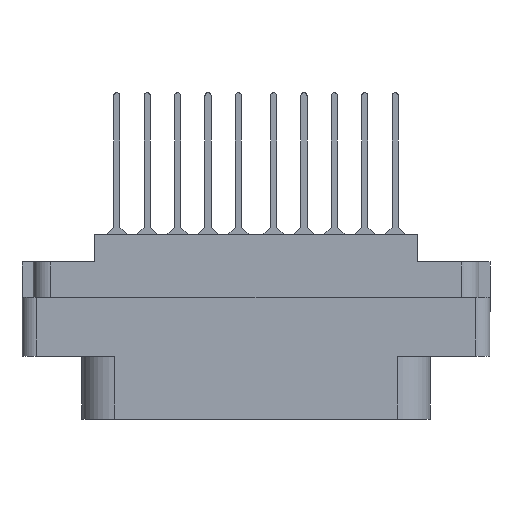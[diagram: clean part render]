
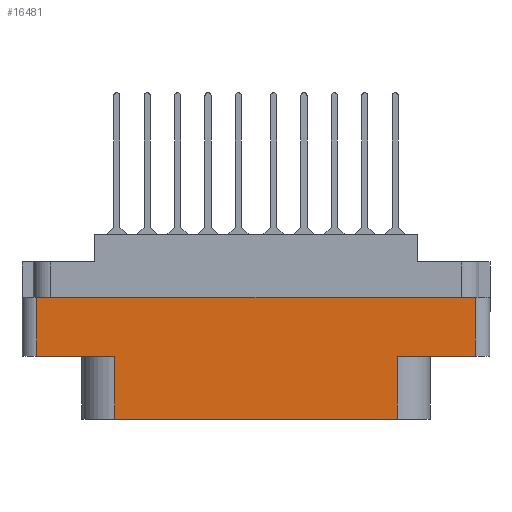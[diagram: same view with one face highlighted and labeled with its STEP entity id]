
A CAD part, front view. The second image highlights one B-rep face of the part: STEP entity #16481.
In plain terms, the highlighted planar face has unit normal (0, -1, 0).
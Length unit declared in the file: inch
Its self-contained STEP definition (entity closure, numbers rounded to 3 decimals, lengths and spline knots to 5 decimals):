
#424 = VECTOR ( 'NONE', #13086, 39.37008 ) ;
#2172 = CARTESIAN_POINT ( 'NONE',  ( 0.938, -0.438, -0.52 ) ) ;
#2329 = CARTESIAN_POINT ( 'NONE',  ( -0.604, -0.438, -0.789 ) ) ;
#3349 = LINE ( 'NONE', #35935, #7940 ) ;
#3606 = EDGE_CURVE ( 'NONE', #11798, #6598, #30297, .T. ) ;
#4166 = CARTESIAN_POINT ( 'NONE',  ( -0.938, -0.438, -0.789 ) ) ;
#5817 = VECTOR ( 'NONE', #22901, 39.37008 ) ;
#6598 = VERTEX_POINT ( 'NONE', #17969 ) ;
#6996 = LINE ( 'NONE', #27918, #11958 ) ;
#7242 = FACE_OUTER_BOUND ( 'NONE', #15127, .T. ) ;
#7872 = VERTEX_POINT ( 'NONE', #2329 ) ;
#7940 = VECTOR ( 'NONE', #24107, 39.37008 ) ;
#8310 = VECTOR ( 'NONE', #18949, 39.37008 ) ;
#10467 = DIRECTION ( 'NONE',  ( 1., 0., 0. ) ) ;
#10650 = DIRECTION ( 'NONE',  ( 1., 0., 0. ) ) ;
#11186 = LINE ( 'NONE', #19456, #34420 ) ;
#11798 = VERTEX_POINT ( 'NONE', #2172 ) ;
#11958 = VECTOR ( 'NONE', #10467, 39.37008 ) ;
#12614 = DIRECTION ( 'NONE',  ( 0., 0., -1. ) ) ;
#13086 = DIRECTION ( 'NONE',  ( 0., 0., -1. ) ) ;
#13253 = EDGE_CURVE ( 'NONE', #30960, #36560, #23623, .T. ) ;
#13269 = ORIENTED_EDGE ( 'NONE', *, *, #32429, .T. ) ;
#15127 = EDGE_LOOP ( 'NONE', ( #34025, #35011, #32678, #32936, #24844, #15879, #19700, #13269 ) ) ;
#15879 = ORIENTED_EDGE ( 'NONE', *, *, #31851, .T. ) ;
#16081 = VECTOR ( 'NONE', #28168, 39.37008 ) ;
#16481 = ADVANCED_FACE ( 'NONE', ( #7242 ), #27015, .T. ) ;
#17959 = VECTOR ( 'NONE', #33594, 39.37008 ) ;
#17969 = CARTESIAN_POINT ( 'NONE',  ( 0.604, -0.438, -0.52 ) ) ;
#18949 = DIRECTION ( 'NONE',  ( 0., 0., 1. ) ) ;
#19183 = CARTESIAN_POINT ( 'NONE',  ( 0.938, -0.438, -0.268 ) ) ;
#19456 = CARTESIAN_POINT ( 'NONE',  ( -1., -0.438, -0.789 ) ) ;
#19700 = ORIENTED_EDGE ( 'NONE', *, *, #3606, .F. ) ;
#21545 = CARTESIAN_POINT ( 'NONE',  ( 0.604, -0.438, -0.789 ) ) ;
#21825 = EDGE_CURVE ( 'NONE', #22371, #7872, #3349, .T. ) ;
#22371 = VERTEX_POINT ( 'NONE', #23176 ) ;
#22901 = DIRECTION ( 'NONE',  ( 1., 0., 0. ) ) ;
#23176 = CARTESIAN_POINT ( 'NONE',  ( -0.604, -0.438, -0.52 ) ) ;
#23623 = LINE ( 'NONE', #4166, #424 ) ;
#24107 = DIRECTION ( 'NONE',  ( 0., 0., -1. ) ) ;
#24844 = ORIENTED_EDGE ( 'NONE', *, *, #29118, .T. ) ;
#25435 = VERTEX_POINT ( 'NONE', #19183 ) ;
#26090 = EDGE_CURVE ( 'NONE', #36560, #22371, #36759, .T. ) ;
#26531 = LINE ( 'NONE', #33713, #8310 ) ;
#27015 = PLANE ( 'NONE',  #27955 ) ;
#27269 = CARTESIAN_POINT ( 'NONE',  ( -1., -0.438, -0.789 ) ) ;
#27312 = VERTEX_POINT ( 'NONE', #21545 ) ;
#27918 = CARTESIAN_POINT ( 'NONE',  ( 0., -0.438, -0.268 ) ) ;
#27955 = AXIS2_PLACEMENT_3D ( 'NONE', #27269, #32864, #12614 ) ;
#28168 = DIRECTION ( 'NONE',  ( 0., 0., 1. ) ) ;
#29118 = EDGE_CURVE ( 'NONE', #7872, #27312, #11186, .T. ) ;
#30297 = LINE ( 'NONE', #30943, #17959 ) ;
#30943 = CARTESIAN_POINT ( 'NONE',  ( 0., -0.438, -0.52 ) ) ;
#30960 = VERTEX_POINT ( 'NONE', #33494 ) ;
#31656 = EDGE_CURVE ( 'NONE', #30960, #25435, #6996, .T. ) ;
#31851 = EDGE_CURVE ( 'NONE', #27312, #6598, #35640, .T. ) ;
#31983 = CARTESIAN_POINT ( 'NONE',  ( 0., -0.438, -0.52 ) ) ;
#32429 = EDGE_CURVE ( 'NONE', #11798, #25435, #26531, .T. ) ;
#32678 = ORIENTED_EDGE ( 'NONE', *, *, #26090, .T. ) ;
#32864 = DIRECTION ( 'NONE',  ( 0., -1., 0. ) ) ;
#32936 = ORIENTED_EDGE ( 'NONE', *, *, #21825, .T. ) ;
#33494 = CARTESIAN_POINT ( 'NONE',  ( -0.938, -0.438, -0.268 ) ) ;
#33594 = DIRECTION ( 'NONE',  ( -1., 0., 0. ) ) ;
#33713 = CARTESIAN_POINT ( 'NONE',  ( 0.938, -0.438, -0.789 ) ) ;
#34025 = ORIENTED_EDGE ( 'NONE', *, *, #31656, .F. ) ;
#34420 = VECTOR ( 'NONE', #10650, 39.37008 ) ;
#35011 = ORIENTED_EDGE ( 'NONE', *, *, #13253, .T. ) ;
#35640 = LINE ( 'NONE', #37276, #16081 ) ;
#35935 = CARTESIAN_POINT ( 'NONE',  ( -0.604, -0.438, -0.789 ) ) ;
#36449 = CARTESIAN_POINT ( 'NONE',  ( -0.938, -0.438, -0.52 ) ) ;
#36560 = VERTEX_POINT ( 'NONE', #36449 ) ;
#36759 = LINE ( 'NONE', #31983, #5817 ) ;
#37276 = CARTESIAN_POINT ( 'NONE',  ( 0.604, -0.438, -0.52 ) ) ;
